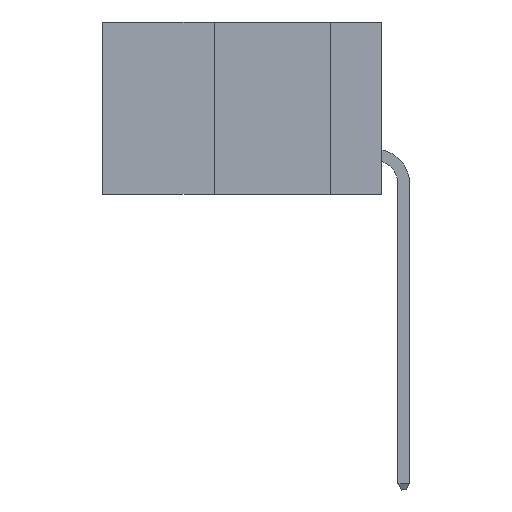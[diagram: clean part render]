
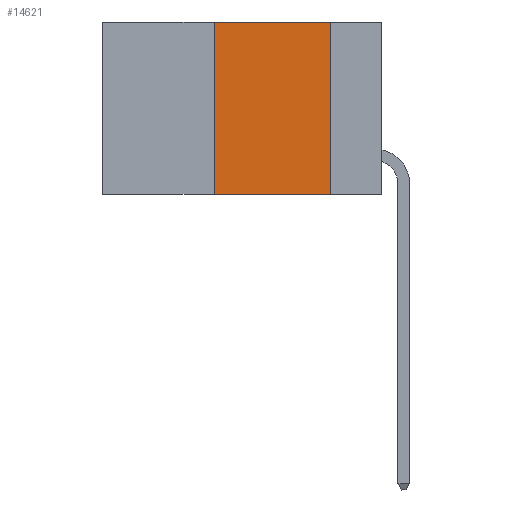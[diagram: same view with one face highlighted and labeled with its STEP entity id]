
A CAD part, left-side view. The second image highlights one B-rep face of the part: STEP entity #14621.
In plain terms, the highlighted planar face has unit normal (-1, 0, 0).
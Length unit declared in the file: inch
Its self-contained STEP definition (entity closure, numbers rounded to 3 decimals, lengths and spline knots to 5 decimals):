
#1101 = CARTESIAN_POINT ( 'NONE',  ( 0., 0.6, 0. ) ) ;
#1109 = CARTESIAN_POINT ( 'NONE',  ( 0., 0.11, 0. ) ) ;
#1819 = CARTESIAN_POINT ( 'NONE',  ( 0., 0.6, 0. ) ) ;
#3021 = DIRECTION ( 'NONE',  ( 0., 0., -1. ) ) ;
#3761 = DIRECTION ( 'NONE',  ( 0., -1., 0. ) ) ;
#4071 = VERTEX_POINT ( 'NONE', #20520 ) ;
#4169 = FACE_OUTER_BOUND ( 'NONE', #15612, .T. ) ;
#4900 = EDGE_CURVE ( 'NONE', #18902, #16102, #5014, .T. ) ;
#5014 = LINE ( 'NONE', #6363, #19877 ) ;
#5856 = VECTOR ( 'NONE', #11146, 39.37008 ) ;
#6363 = CARTESIAN_POINT ( 'NONE',  ( 0., 0.11, 0. ) ) ;
#7082 = AXIS2_PLACEMENT_3D ( 'NONE', #1101, #14649, #3021 ) ;
#9272 = VERTEX_POINT ( 'NONE', #20498 ) ;
#9330 = LINE ( 'NONE', #23616, #19024 ) ;
#10117 = CARTESIAN_POINT ( 'NONE',  ( 0., 0.11, -0.37 ) ) ;
#10829 = EDGE_CURVE ( 'NONE', #9272, #18902, #18056, .T. ) ;
#10994 = LINE ( 'NONE', #13070, #5856 ) ;
#11146 = DIRECTION ( 'NONE',  ( 0., 0., 1. ) ) ;
#12076 = DIRECTION ( 'NONE',  ( 0., 0., -1. ) ) ;
#12845 = VECTOR ( 'NONE', #3761, 39.37008 ) ;
#13070 = CARTESIAN_POINT ( 'NONE',  ( 0., 0.36, 0. ) ) ;
#13153 = ORIENTED_EDGE ( 'NONE', *, *, #10829, .F. ) ;
#14007 = DIRECTION ( 'NONE',  ( 0., -1., 0. ) ) ;
#14621 = ADVANCED_FACE ( 'NONE', ( #4169 ), #20437, .F. ) ;
#14649 = DIRECTION ( 'NONE',  ( 1., 0., 0. ) ) ;
#15080 = EDGE_CURVE ( 'NONE', #4071, #16102, #9330, .T. ) ;
#15612 = EDGE_LOOP ( 'NONE', ( #21370, #13153, #22276, #21681 ) ) ;
#16102 = VERTEX_POINT ( 'NONE', #10117 ) ;
#18056 = LINE ( 'NONE', #1819, #12845 ) ;
#18902 = VERTEX_POINT ( 'NONE', #1109 ) ;
#19024 = VECTOR ( 'NONE', #14007, 39.37008 ) ;
#19877 = VECTOR ( 'NONE', #12076, 39.37008 ) ;
#20437 = PLANE ( 'NONE',  #7082 ) ;
#20498 = CARTESIAN_POINT ( 'NONE',  ( 0., 0.36, 0. ) ) ;
#20520 = CARTESIAN_POINT ( 'NONE',  ( 0., 0.36, -0.37 ) ) ;
#21370 = ORIENTED_EDGE ( 'NONE', *, *, #4900, .F. ) ;
#21681 = ORIENTED_EDGE ( 'NONE', *, *, #15080, .T. ) ;
#22276 = ORIENTED_EDGE ( 'NONE', *, *, #24729, .F. ) ;
#23616 = CARTESIAN_POINT ( 'NONE',  ( 0., 0.6, -0.37 ) ) ;
#24729 = EDGE_CURVE ( 'NONE', #4071, #9272, #10994, .T. ) ;
